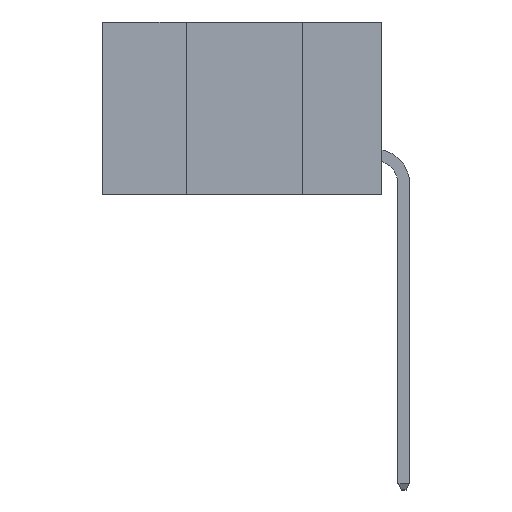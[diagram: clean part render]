
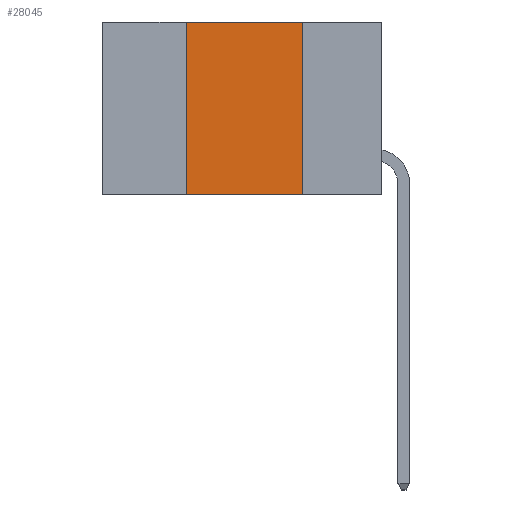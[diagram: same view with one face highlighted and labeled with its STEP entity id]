
A CAD part, left-side view. The second image highlights one B-rep face of the part: STEP entity #28045.
In plain terms, the highlighted planar face has unit normal (-1, 0, 0).
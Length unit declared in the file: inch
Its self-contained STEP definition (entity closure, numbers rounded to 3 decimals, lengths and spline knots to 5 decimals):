
#1450 = CARTESIAN_POINT ( 'NONE',  ( 0., 0.17, -0.37 ) ) ;
#2798 = VERTEX_POINT ( 'NONE', #1450 ) ;
#5170 = LINE ( 'NONE', #8340, #16643 ) ;
#8340 = CARTESIAN_POINT ( 'NONE',  ( 0., 0.6, -0.37 ) ) ;
#9680 = DIRECTION ( 'NONE',  ( 0., 0., -1. ) ) ;
#10713 = CARTESIAN_POINT ( 'NONE',  ( 0., 0.42, -0.37 ) ) ;
#12559 = CARTESIAN_POINT ( 'NONE',  ( 0., 0.42, 0. ) ) ;
#12612 = EDGE_CURVE ( 'NONE', #41245, #36696, #22398, .T. ) ;
#13592 = DIRECTION ( 'NONE',  ( 0., 0., -1. ) ) ;
#16536 = EDGE_CURVE ( 'NONE', #36696, #38668, #24499, .T. ) ;
#16643 = VECTOR ( 'NONE', #34356, 39.37008 ) ;
#17159 = CARTESIAN_POINT ( 'NONE',  ( 0., 0.17, 0. ) ) ;
#19124 = PLANE ( 'NONE',  #30977 ) ;
#20357 = EDGE_CURVE ( 'NONE', #38668, #2798, #39835, .T. ) ;
#22267 = VECTOR ( 'NONE', #13592, 39.37008 ) ;
#22398 = LINE ( 'NONE', #31633, #23431 ) ;
#23431 = VECTOR ( 'NONE', #37939, 39.37008 ) ;
#23671 = CARTESIAN_POINT ( 'NONE',  ( 0., 0.17, 0. ) ) ;
#24499 = LINE ( 'NONE', #33326, #36439 ) ;
#28045 = ADVANCED_FACE ( 'NONE', ( #40955 ), #19124, .F. ) ;
#28700 = ORIENTED_EDGE ( 'NONE', *, *, #37450, .T. ) ;
#30977 = AXIS2_PLACEMENT_3D ( 'NONE', #31726, #37593, #9680 ) ;
#31633 = CARTESIAN_POINT ( 'NONE',  ( 0., 0.42, 0. ) ) ;
#31726 = CARTESIAN_POINT ( 'NONE',  ( 0., 0.6, 0. ) ) ;
#32511 = ORIENTED_EDGE ( 'NONE', *, *, #20357, .F. ) ;
#33326 = CARTESIAN_POINT ( 'NONE',  ( 0., 0.6, 0. ) ) ;
#34142 = DIRECTION ( 'NONE',  ( 0., -1., 0. ) ) ;
#34356 = DIRECTION ( 'NONE',  ( 0., -1., 0. ) ) ;
#36439 = VECTOR ( 'NONE', #34142, 39.37008 ) ;
#36696 = VERTEX_POINT ( 'NONE', #12559 ) ;
#37450 = EDGE_CURVE ( 'NONE', #41245, #2798, #5170, .T. ) ;
#37593 = DIRECTION ( 'NONE',  ( 1., 0., 0. ) ) ;
#37939 = DIRECTION ( 'NONE',  ( 0., 0., 1. ) ) ;
#38312 = ORIENTED_EDGE ( 'NONE', *, *, #16536, .F. ) ;
#38668 = VERTEX_POINT ( 'NONE', #23671 ) ;
#39244 = ORIENTED_EDGE ( 'NONE', *, *, #12612, .F. ) ;
#39295 = EDGE_LOOP ( 'NONE', ( #32511, #38312, #39244, #28700 ) ) ;
#39835 = LINE ( 'NONE', #17159, #22267 ) ;
#40955 = FACE_OUTER_BOUND ( 'NONE', #39295, .T. ) ;
#41245 = VERTEX_POINT ( 'NONE', #10713 ) ;
